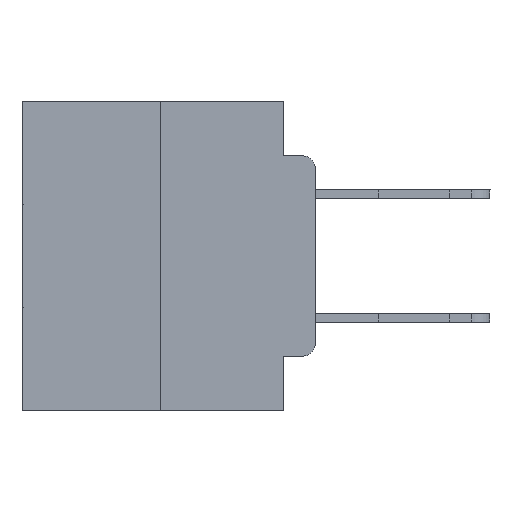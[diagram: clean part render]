
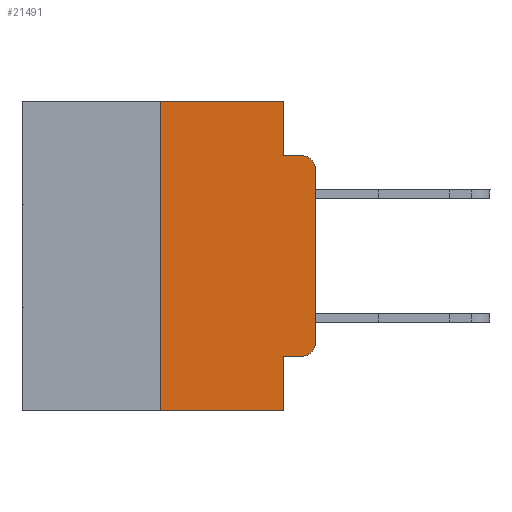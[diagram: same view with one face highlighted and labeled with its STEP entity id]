
A CAD part, left-side view. The second image highlights one B-rep face of the part: STEP entity #21491.
In plain terms, the highlighted planar face has unit normal (-1, 0, 0).
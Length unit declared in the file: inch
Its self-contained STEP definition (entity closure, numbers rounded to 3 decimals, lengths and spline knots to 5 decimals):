
#85 = VERTEX_POINT ( 'NONE', #4651 ) ;
#2064 = AXIS2_PLACEMENT_3D ( 'NONE', #9583, #26747, #7496 ) ;
#3401 = CARTESIAN_POINT ( 'NONE',  ( 0., 0.051, -0.0885 ) ) ;
#3438 = ORIENTED_EDGE ( 'NONE', *, *, #26562, .T. ) ;
#4167 = LINE ( 'NONE', #21448, #20813 ) ;
#4234 = EDGE_CURVE ( 'NONE', #6410, #27652, #7959, .T. ) ;
#4516 = CARTESIAN_POINT ( 'NONE',  ( 0., 0.051, 0. ) ) ;
#4610 = FACE_OUTER_BOUND ( 'NONE', #16773, .T. ) ;
#4651 = CARTESIAN_POINT ( 'NONE',  ( 0., 0.051, 0. ) ) ;
#4713 = CARTESIAN_POINT ( 'NONE',  ( 0., 0.051, -0.5 ) ) ;
#4805 = EDGE_CURVE ( 'NONE', #16542, #27652, #23778, .T. ) ;
#5439 = VECTOR ( 'NONE', #16491, 39.37008 ) ;
#5556 = CARTESIAN_POINT ( 'NONE',  ( 0., 0.473, -0.5 ) ) ;
#5671 = EDGE_CURVE ( 'NONE', #16439, #21999, #4167, .T. ) ;
#6410 = VERTEX_POINT ( 'NONE', #26285 ) ;
#6446 = DIRECTION ( 'NONE',  ( 1., 0., 0. ) ) ;
#6451 = VECTOR ( 'NONE', #11002, 39.37008 ) ;
#7496 = DIRECTION ( 'NONE',  ( 0., 0., -1. ) ) ;
#7959 = LINE ( 'NONE', #5556, #5439 ) ;
#7982 = DIRECTION ( 'NONE',  ( -1., 0., 0. ) ) ;
#8627 = VERTEX_POINT ( 'NONE', #26079 ) ;
#8772 = CIRCLE ( 'NONE', #19530, 0.02 ) ;
#8856 = VERTEX_POINT ( 'NONE', #22399 ) ;
#9273 = DIRECTION ( 'NONE',  ( 0., 0., 1. ) ) ;
#9583 = CARTESIAN_POINT ( 'NONE',  ( 0., 0.02, -0.1085 ) ) ;
#11002 = DIRECTION ( 'NONE',  ( 0., -1., 0. ) ) ;
#11559 = LINE ( 'NONE', #20131, #15651 ) ;
#12632 = AXIS2_PLACEMENT_3D ( 'NONE', #21904, #6446, #12909 ) ;
#12881 = CARTESIAN_POINT ( 'NONE',  ( 0., 0.02, -0.3915 ) ) ;
#12909 = DIRECTION ( 'NONE',  ( 0., 0., -1. ) ) ;
#12959 = EDGE_CURVE ( 'NONE', #85, #16439, #16843, .T. ) ;
#13122 = ORIENTED_EDGE ( 'NONE', *, *, #17693, .T. ) ;
#13184 = ORIENTED_EDGE ( 'NONE', *, *, #5671, .F. ) ;
#13244 = CARTESIAN_POINT ( 'NONE',  ( 0., 0.473, 0. ) ) ;
#13996 = CARTESIAN_POINT ( 'NONE',  ( 0., 0.02, -0.0885 ) ) ;
#14763 = CARTESIAN_POINT ( 'NONE',  ( 0., 0.051, -0.4115 ) ) ;
#14895 = ORIENTED_EDGE ( 'NONE', *, *, #23960, .F. ) ;
#15432 = ORIENTED_EDGE ( 'NONE', *, *, #26461, .T. ) ;
#15439 = VECTOR ( 'NONE', #9273, 39.37008 ) ;
#15651 = VECTOR ( 'NONE', #16433, 39.37008 ) ;
#15997 = ORIENTED_EDGE ( 'NONE', *, *, #4805, .F. ) ;
#16031 = ORIENTED_EDGE ( 'NONE', *, *, #4234, .T. ) ;
#16165 = ORIENTED_EDGE ( 'NONE', *, *, #12959, .F. ) ;
#16433 = DIRECTION ( 'NONE',  ( 0., 0., 1. ) ) ;
#16439 = VERTEX_POINT ( 'NONE', #3401 ) ;
#16491 = DIRECTION ( 'NONE',  ( 0., -1., 0. ) ) ;
#16542 = VERTEX_POINT ( 'NONE', #23616 ) ;
#16773 = EDGE_LOOP ( 'NONE', ( #13122, #15432, #13184, #16165, #14895, #24058, #16031, #15997, #3438, #20973 ) ) ;
#16843 = LINE ( 'NONE', #23994, #24996 ) ;
#16858 = DIRECTION ( 'NONE',  ( 0., -1., 0. ) ) ;
#17516 = DIRECTION ( 'NONE',  ( 0., 0., -1. ) ) ;
#17693 = EDGE_CURVE ( 'NONE', #21902, #8627, #11559, .T. ) ;
#17967 = CARTESIAN_POINT ( 'NONE',  ( 0., 0.25, 0. ) ) ;
#19530 = AXIS2_PLACEMENT_3D ( 'NONE', #12881, #7982, #27241 ) ;
#20131 = CARTESIAN_POINT ( 'NONE',  ( 0., 0., 0. ) ) ;
#20813 = VECTOR ( 'NONE', #21589, 39.37008 ) ;
#20973 = ORIENTED_EDGE ( 'NONE', *, *, #27436, .T. ) ;
#21288 = VECTOR ( 'NONE', #25907, 39.37008 ) ;
#21444 = CARTESIAN_POINT ( 'NONE',  ( 0., 0., -0.3915 ) ) ;
#21448 = CARTESIAN_POINT ( 'NONE',  ( 0., 0.051, -0.0885 ) ) ;
#21491 = ADVANCED_FACE ( 'NONE', ( #4610 ), #21624, .F. ) ;
#21589 = DIRECTION ( 'NONE',  ( 0., -1., 0. ) ) ;
#21624 = PLANE ( 'NONE',  #12632 ) ;
#21902 = VERTEX_POINT ( 'NONE', #21444 ) ;
#21904 = CARTESIAN_POINT ( 'NONE',  ( 0., 0.473, 0. ) ) ;
#21999 = VERTEX_POINT ( 'NONE', #13996 ) ;
#22300 = VERTEX_POINT ( 'NONE', #23825 ) ;
#22399 = CARTESIAN_POINT ( 'NONE',  ( 0., 0.25, 0. ) ) ;
#23616 = CARTESIAN_POINT ( 'NONE',  ( 0., 0.051, -0.4115 ) ) ;
#23778 = LINE ( 'NONE', #4516, #21288 ) ;
#23825 = CARTESIAN_POINT ( 'NONE',  ( 0., 0.02, -0.4115 ) ) ;
#23960 = EDGE_CURVE ( 'NONE', #8856, #85, #24067, .T. ) ;
#23994 = CARTESIAN_POINT ( 'NONE',  ( 0., 0.051, 0. ) ) ;
#24058 = ORIENTED_EDGE ( 'NONE', *, *, #24516, .F. ) ;
#24067 = LINE ( 'NONE', #13244, #6451 ) ;
#24516 = EDGE_CURVE ( 'NONE', #6410, #8856, #26438, .T. ) ;
#24538 = VECTOR ( 'NONE', #16858, 39.37008 ) ;
#24996 = VECTOR ( 'NONE', #17516, 39.37008 ) ;
#25869 = CIRCLE ( 'NONE', #2064, 0.02 ) ;
#25907 = DIRECTION ( 'NONE',  ( 0., 0., -1. ) ) ;
#26079 = CARTESIAN_POINT ( 'NONE',  ( 0., 0., -0.1085 ) ) ;
#26285 = CARTESIAN_POINT ( 'NONE',  ( 0., 0.25, -0.5 ) ) ;
#26438 = LINE ( 'NONE', #17967, #15439 ) ;
#26461 = EDGE_CURVE ( 'NONE', #8627, #21999, #25869, .T. ) ;
#26562 = EDGE_CURVE ( 'NONE', #16542, #22300, #27576, .T. ) ;
#26747 = DIRECTION ( 'NONE',  ( -1., 0., 0. ) ) ;
#27241 = DIRECTION ( 'NONE',  ( 0., 0., -1. ) ) ;
#27436 = EDGE_CURVE ( 'NONE', #22300, #21902, #8772, .T. ) ;
#27576 = LINE ( 'NONE', #14763, #24538 ) ;
#27652 = VERTEX_POINT ( 'NONE', #4713 ) ;
